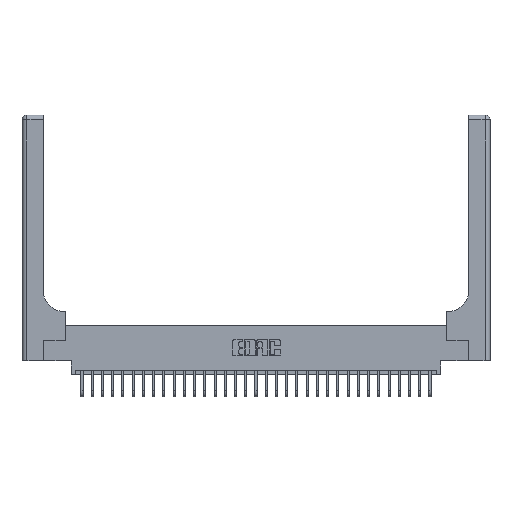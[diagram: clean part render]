
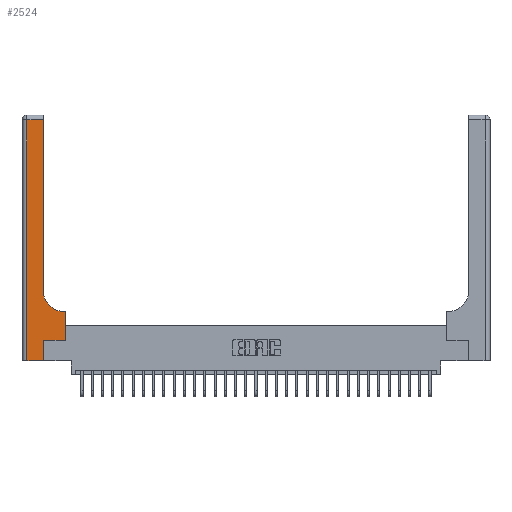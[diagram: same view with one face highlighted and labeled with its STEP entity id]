
A CAD part, top view. The second image highlights one B-rep face of the part: STEP entity #2524.
In plain terms, the highlighted planar face has unit normal (0, 0, 1).
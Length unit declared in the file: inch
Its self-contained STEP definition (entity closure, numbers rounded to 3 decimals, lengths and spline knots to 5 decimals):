
#1120 = VECTOR ( 'NONE', #26243, 39.37008 ) ;
#1310 = CARTESIAN_POINT ( 'NONE',  ( 0.265, 0.25, 0.37 ) ) ;
#1551 = VECTOR ( 'NONE', #12547, 39.37008 ) ;
#1559 = ORIENTED_EDGE ( 'NONE', *, *, #15870, .T. ) ;
#1791 = ORIENTED_EDGE ( 'NONE', *, *, #27875, .T. ) ;
#1838 = ORIENTED_EDGE ( 'NONE', *, *, #20440, .T. ) ;
#2524 = ADVANCED_FACE ( 'NONE', ( #19602 ), #18972, .F. ) ;
#4110 = LINE ( 'NONE', #9895, #12706 ) ;
#4761 = CIRCLE ( 'NONE', #4809, 0.25 ) ;
#4809 = AXIS2_PLACEMENT_3D ( 'NONE', #30271, #30469, #18156 ) ;
#5335 = VECTOR ( 'NONE', #11693, 39.37008 ) ;
#5394 = EDGE_CURVE ( 'NONE', #8748, #7353, #11991, .T. ) ;
#5541 = CARTESIAN_POINT ( 'NONE',  ( 0.26, 2.94, 0.37 ) ) ;
#6656 = CARTESIAN_POINT ( 'NONE',  ( 0.528, 0.6, 0.37 ) ) ;
#6825 = CARTESIAN_POINT ( 'NONE',  ( 0.26, 0.6, 0.37 ) ) ;
#6893 = CARTESIAN_POINT ( 'NONE',  ( 0., 0., 0.37 ) ) ;
#7255 = EDGE_CURVE ( 'NONE', #22818, #23230, #16821, .T. ) ;
#7353 = VERTEX_POINT ( 'NONE', #11728 ) ;
#8748 = VERTEX_POINT ( 'NONE', #6656 ) ;
#9154 = CARTESIAN_POINT ( 'NONE',  ( 0., 2.94, 0.37 ) ) ;
#9230 = DIRECTION ( 'NONE',  ( -1., 0., 0. ) ) ;
#9239 = DIRECTION ( 'NONE',  ( 0., 0., -1. ) ) ;
#9814 = VERTEX_POINT ( 'NONE', #10864 ) ;
#9895 = CARTESIAN_POINT ( 'NONE',  ( 0.528, 0.25, 0.37 ) ) ;
#10084 = DIRECTION ( 'NONE',  ( 0., 1., 0. ) ) ;
#10452 = VECTOR ( 'NONE', #9230, 39.37008 ) ;
#10864 = CARTESIAN_POINT ( 'NONE',  ( 0.528, 0.25, 0.37 ) ) ;
#11693 = DIRECTION ( 'NONE',  ( -1., 0., 0. ) ) ;
#11728 = CARTESIAN_POINT ( 'NONE',  ( 0.51, 0.6, 0.37 ) ) ;
#11991 = LINE ( 'NONE', #6825, #10452 ) ;
#12491 = CARTESIAN_POINT ( 'NONE',  ( 0.06, 3., 0.37 ) ) ;
#12547 = DIRECTION ( 'NONE',  ( 0., 1., 0. ) ) ;
#12593 = CARTESIAN_POINT ( 'NONE',  ( 0.06, 2.94, 0.37 ) ) ;
#12706 = VECTOR ( 'NONE', #10084, 39.37008 ) ;
#12757 = CARTESIAN_POINT ( 'NONE',  ( 0.265, 0., 0.37 ) ) ;
#12891 = EDGE_CURVE ( 'NONE', #23230, #14292, #25471, .T. ) ;
#13377 = ORIENTED_EDGE ( 'NONE', *, *, #7255, .T. ) ;
#13658 = EDGE_CURVE ( 'NONE', #13670, #16622, #27689, .T. ) ;
#13670 = VERTEX_POINT ( 'NONE', #21671 ) ;
#14292 = VERTEX_POINT ( 'NONE', #28738 ) ;
#14582 = DIRECTION ( 'NONE',  ( 0., 1., 0. ) ) ;
#14724 = ORIENTED_EDGE ( 'NONE', *, *, #13658, .T. ) ;
#15401 = DIRECTION ( 'NONE',  ( 1., 0., 0. ) ) ;
#15789 = VECTOR ( 'NONE', #15401, 39.37008 ) ;
#15870 = EDGE_CURVE ( 'NONE', #9814, #8748, #4110, .T. ) ;
#16265 = ORIENTED_EDGE ( 'NONE', *, *, #12891, .T. ) ;
#16567 = EDGE_LOOP ( 'NONE', ( #14724, #1838, #28366, #13377, #16265, #30388, #1559, #21552, #1791 ) ) ;
#16622 = VERTEX_POINT ( 'NONE', #5541 ) ;
#16821 = LINE ( 'NONE', #6893, #1120 ) ;
#17093 = DIRECTION ( 'NONE',  ( 0., -1., 0. ) ) ;
#18156 = DIRECTION ( 'NONE',  ( 1., 0., 0. ) ) ;
#18411 = LINE ( 'NONE', #1310, #15789 ) ;
#18723 = VECTOR ( 'NONE', #14582, 39.37008 ) ;
#18860 = EDGE_CURVE ( 'NONE', #20731, #22818, #30852, .T. ) ;
#18972 = PLANE ( 'NONE',  #20677 ) ;
#19574 = LINE ( 'NONE', #9154, #5335 ) ;
#19602 = FACE_OUTER_BOUND ( 'NONE', #16567, .T. ) ;
#20249 = CARTESIAN_POINT ( 'NONE',  ( 0.265, 0., 0.37 ) ) ;
#20440 = EDGE_CURVE ( 'NONE', #16622, #20731, #19574, .T. ) ;
#20677 = AXIS2_PLACEMENT_3D ( 'NONE', #28284, #9239, #23685 ) ;
#20731 = VERTEX_POINT ( 'NONE', #12593 ) ;
#21552 = ORIENTED_EDGE ( 'NONE', *, *, #5394, .T. ) ;
#21671 = CARTESIAN_POINT ( 'NONE',  ( 0.26, 0.85, 0.37 ) ) ;
#22031 = EDGE_CURVE ( 'NONE', #14292, #9814, #18411, .T. ) ;
#22818 = VERTEX_POINT ( 'NONE', #25832 ) ;
#22855 = CARTESIAN_POINT ( 'NONE',  ( 0.26, 3., 0.37 ) ) ;
#23230 = VERTEX_POINT ( 'NONE', #20249 ) ;
#23685 = DIRECTION ( 'NONE',  ( -1., 0., 0. ) ) ;
#23766 = VECTOR ( 'NONE', #17093, 39.37008 ) ;
#25471 = LINE ( 'NONE', #12757, #1551 ) ;
#25832 = CARTESIAN_POINT ( 'NONE',  ( 0.06, 0., 0.37 ) ) ;
#26243 = DIRECTION ( 'NONE',  ( 1., 0., 0. ) ) ;
#27689 = LINE ( 'NONE', #22855, #18723 ) ;
#27875 = EDGE_CURVE ( 'NONE', #7353, #13670, #4761, .T. ) ;
#28284 = CARTESIAN_POINT ( 'NONE',  ( 0., 3., 0.37 ) ) ;
#28366 = ORIENTED_EDGE ( 'NONE', *, *, #18860, .T. ) ;
#28738 = CARTESIAN_POINT ( 'NONE',  ( 0.265, 0.25, 0.37 ) ) ;
#30271 = CARTESIAN_POINT ( 'NONE',  ( 0.51, 0.85, 0.37 ) ) ;
#30388 = ORIENTED_EDGE ( 'NONE', *, *, #22031, .T. ) ;
#30469 = DIRECTION ( 'NONE',  ( 0., 0., -1. ) ) ;
#30852 = LINE ( 'NONE', #12491, #23766 ) ;
